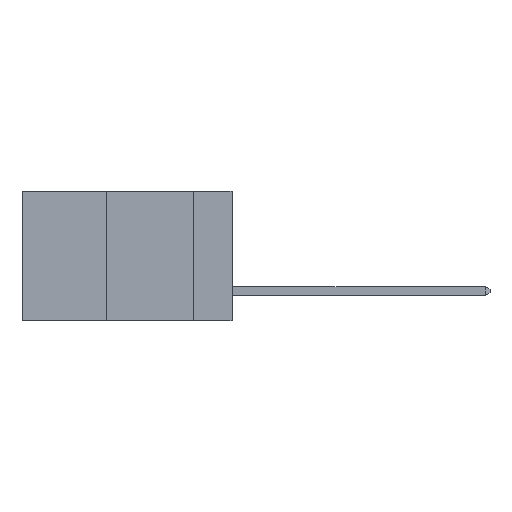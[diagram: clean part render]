
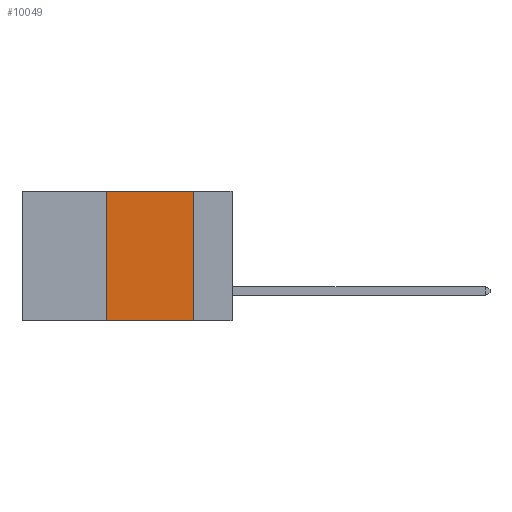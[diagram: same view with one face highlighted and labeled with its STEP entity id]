
A CAD part, left-side view. The second image highlights one B-rep face of the part: STEP entity #10049.
In plain terms, the highlighted planar face has unit normal (-1, 0, 0).
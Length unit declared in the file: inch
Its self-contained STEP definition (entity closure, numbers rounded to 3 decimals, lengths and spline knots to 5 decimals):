
#804 = DIRECTION ( 'NONE',  ( 0., -1., 0. ) ) ;
#1302 = VECTOR ( 'NONE', #19898, 39.37008 ) ;
#1352 = VECTOR ( 'NONE', #804, 39.37008 ) ;
#1929 = VERTEX_POINT ( 'NONE', #19674 ) ;
#2821 = AXIS2_PLACEMENT_3D ( 'NONE', #25072, #11400, #27412 ) ;
#3578 = VECTOR ( 'NONE', #4944, 39.37008 ) ;
#4533 = CARTESIAN_POINT ( 'NONE',  ( 0., 0.11, -0.37 ) ) ;
#4944 = DIRECTION ( 'NONE',  ( 0., -1., 0. ) ) ;
#5617 = CARTESIAN_POINT ( 'NONE',  ( 0., 0.36, -0.37 ) ) ;
#7822 = EDGE_CURVE ( 'NONE', #9217, #1929, #21138, .T. ) ;
#8553 = CARTESIAN_POINT ( 'NONE',  ( 0., 0.11, 0. ) ) ;
#9033 = ORIENTED_EDGE ( 'NONE', *, *, #26792, .T. ) ;
#9217 = VERTEX_POINT ( 'NONE', #5617 ) ;
#9404 = ORIENTED_EDGE ( 'NONE', *, *, #7822, .F. ) ;
#9902 = CARTESIAN_POINT ( 'NONE',  ( 0., 0.36, 0. ) ) ;
#10049 = ADVANCED_FACE ( 'NONE', ( #11357 ), #22779, .F. ) ;
#10092 = ORIENTED_EDGE ( 'NONE', *, *, #17026, .F. ) ;
#11094 = EDGE_CURVE ( 'NONE', #25308, #18985, #19522, .T. ) ;
#11357 = FACE_OUTER_BOUND ( 'NONE', #25991, .T. ) ;
#11400 = DIRECTION ( 'NONE',  ( 1., 0., 0. ) ) ;
#14346 = VECTOR ( 'NONE', #25873, 39.37008 ) ;
#17026 = EDGE_CURVE ( 'NONE', #1929, #25308, #26409, .T. ) ;
#17440 = ORIENTED_EDGE ( 'NONE', *, *, #11094, .F. ) ;
#18609 = CARTESIAN_POINT ( 'NONE',  ( 0., 0.6, -0.37 ) ) ;
#18985 = VERTEX_POINT ( 'NONE', #4533 ) ;
#19522 = LINE ( 'NONE', #8553, #1302 ) ;
#19674 = CARTESIAN_POINT ( 'NONE',  ( 0., 0.36, 0. ) ) ;
#19898 = DIRECTION ( 'NONE',  ( 0., 0., -1. ) ) ;
#21138 = LINE ( 'NONE', #9902, #14346 ) ;
#22779 = PLANE ( 'NONE',  #2821 ) ;
#25072 = CARTESIAN_POINT ( 'NONE',  ( 0., 0.6, 0. ) ) ;
#25308 = VERTEX_POINT ( 'NONE', #26920 ) ;
#25751 = LINE ( 'NONE', #18609, #3578 ) ;
#25873 = DIRECTION ( 'NONE',  ( 0., 0., 1. ) ) ;
#25991 = EDGE_LOOP ( 'NONE', ( #17440, #10092, #9404, #9033 ) ) ;
#26409 = LINE ( 'NONE', #28249, #1352 ) ;
#26792 = EDGE_CURVE ( 'NONE', #9217, #18985, #25751, .T. ) ;
#26920 = CARTESIAN_POINT ( 'NONE',  ( 0., 0.11, 0. ) ) ;
#27412 = DIRECTION ( 'NONE',  ( 0., 0., -1. ) ) ;
#28249 = CARTESIAN_POINT ( 'NONE',  ( 0., 0.6, 0. ) ) ;
